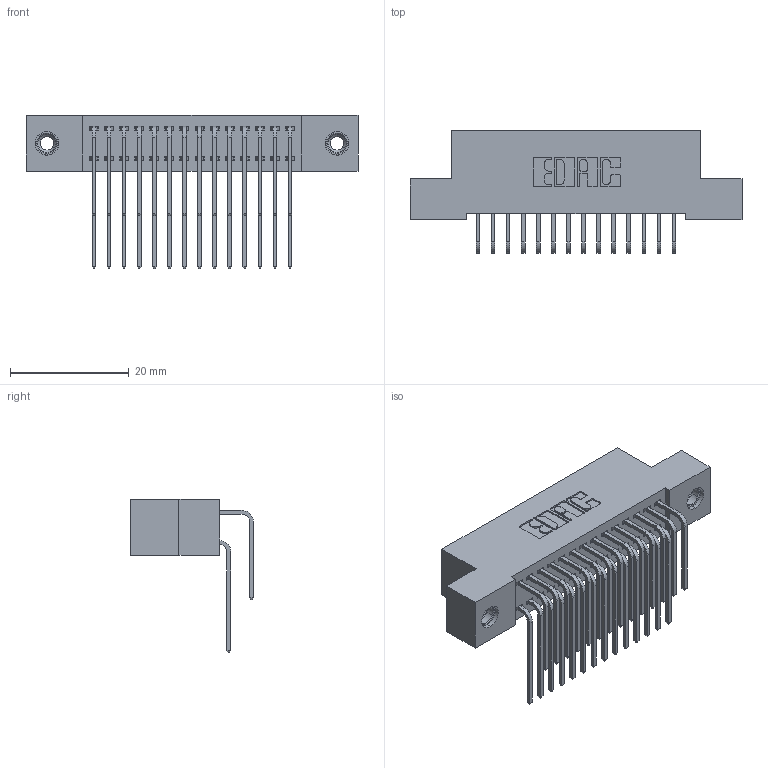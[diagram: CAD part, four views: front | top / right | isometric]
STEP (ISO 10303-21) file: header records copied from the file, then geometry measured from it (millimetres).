
FILE_DESCRIPTION (( 'STEP AP203' ), '1' );
FILE_NAME ('392-028-559-208.STEP', '2018-08-15T21:34:12', ( '' ), ( '' ), 'SwSTEP 2.0', 'SolidWorks 2016', '' );
FILE_SCHEMA (( 'CONFIG_CONTROL_DESIGN' ));
Length unit declared in the file: inch
Products named in the file (5): 345-250-001_345-250-003-102; 392-028-559-208; 342 Part_TI; 345-292-001_558 559 Tail - 1; 345-292-001_559 Tail - 2
Assembly tree (31 placements, depth 2):
  392-028-559-208
    342 Part_TI
    345-292-001_558 559 Tail - 1  x14
    345-292-001_559 Tail - 2  x14
    345-250-001_345-250-003-102  x2
Bounding box: 55.88 x 20.64 x 25.78 mm (x, y, z)
Volume: 5044.1 mm3; surface area: 8261.6 mm2
Topology: 31 solids, 31 shells, 1682 faces, 4943 edges, 3250 vertices
Faces by surface type: plane 1162, cylinder 504, cone 12, torus 4
Entity records: 15466 total; most frequent: CARTESIAN_POINT 2628, ORIENTED_EDGE 2506, DIRECTION 2307, EDGE_CURVE 1253, VECTOR 1065, LINE 1065, VERTEX_POINT 828, AXIS2_PLACEMENT_3D 621
